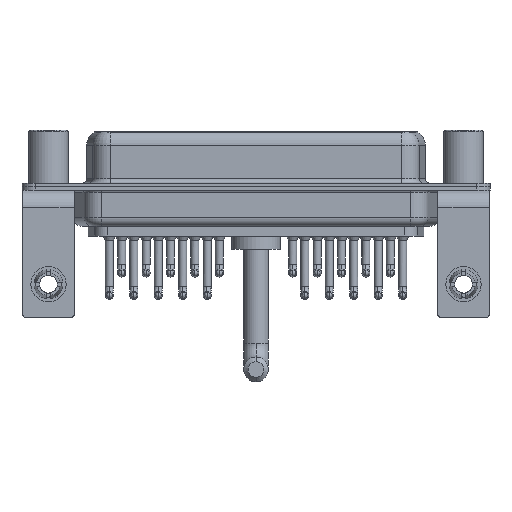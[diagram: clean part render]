
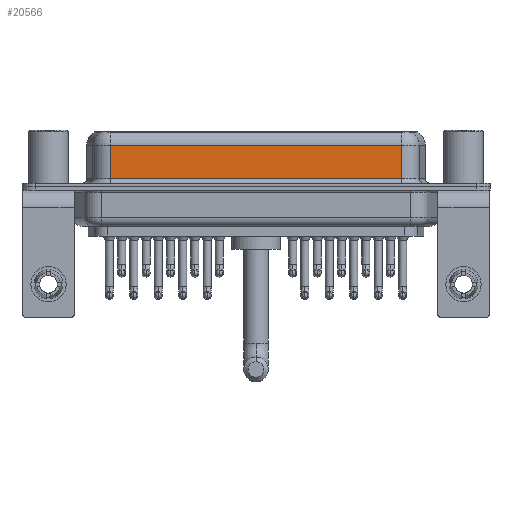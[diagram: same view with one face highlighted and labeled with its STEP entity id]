
A CAD part, front view. The second image highlights one B-rep face of the part: STEP entity #20566.
In plain terms, the highlighted planar face has unit normal (0, -1, 0).
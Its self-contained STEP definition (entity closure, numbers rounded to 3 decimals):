
#22 = DIRECTION ( 'NONE',  ( 0., 0., -1. ) ) ;
#668 = CARTESIAN_POINT ( 'NONE',  ( 40.037, -3.95, 4.65 ) ) ;
#1935 = DIRECTION ( 'NONE',  ( 0., 0., 1. ) ) ;
#2299 = LINE ( 'NONE', #668, #20552 ) ;
#2890 = VECTOR ( 'NONE', #9590, 1000. ) ;
#4066 = VECTOR ( 'NONE', #22, 1000. ) ;
#5206 = EDGE_CURVE ( 'NONE', #19438, #12582, #13756, .T. ) ;
#5814 = ORIENTED_EDGE ( 'NONE', *, *, #12244, .T. ) ;
#5881 = PLANE ( 'NONE',  #21403 ) ;
#9406 = VECTOR ( 'NONE', #24318, 1000. ) ;
#9524 = CARTESIAN_POINT ( 'NONE',  ( 40.037, -3.95, 0.9 ) ) ;
#9590 = DIRECTION ( 'NONE',  ( 0., 0., -1. ) ) ;
#9734 = LINE ( 'NONE', #14180, #2890 ) ;
#9865 = ORIENTED_EDGE ( 'NONE', *, *, #10973, .F. ) ;
#10973 = EDGE_CURVE ( 'NONE', #15545, #12582, #20626, .T. ) ;
#12244 = EDGE_CURVE ( 'NONE', #12977, #19438, #9734, .T. ) ;
#12582 = VERTEX_POINT ( 'NONE', #9524 ) ;
#12977 = VERTEX_POINT ( 'NONE', #15857 ) ;
#13756 = LINE ( 'NONE', #22438, #9406 ) ;
#13770 = ORIENTED_EDGE ( 'NONE', *, *, #5206, .T. ) ;
#14180 = CARTESIAN_POINT ( 'NONE',  ( 7.013, -3.95, 6.4 ) ) ;
#15545 = VERTEX_POINT ( 'NONE', #24174 ) ;
#15857 = CARTESIAN_POINT ( 'NONE',  ( 7.013, -3.95, 4.65 ) ) ;
#18470 = DIRECTION ( 'NONE',  ( 0., 1., 0. ) ) ;
#18867 = CARTESIAN_POINT ( 'NONE',  ( 7.013, -3.95, 0.9 ) ) ;
#19438 = VERTEX_POINT ( 'NONE', #18867 ) ;
#20497 = FACE_OUTER_BOUND ( 'NONE', #20662, .T. ) ;
#20552 = VECTOR ( 'NONE', #20862, 1000. ) ;
#20566 = ADVANCED_FACE ( 'NONE', ( #20497 ), #5881, .F. ) ;
#20626 = LINE ( 'NONE', #25087, #4066 ) ;
#20662 = EDGE_LOOP ( 'NONE', ( #9865, #20981, #5814, #13770 ) ) ;
#20862 = DIRECTION ( 'NONE',  ( -1., 0., 0. ) ) ;
#20895 = CARTESIAN_POINT ( 'NONE',  ( 40.037, -3.95, 6.4 ) ) ;
#20981 = ORIENTED_EDGE ( 'NONE', *, *, #21110, .T. ) ;
#21110 = EDGE_CURVE ( 'NONE', #15545, #12977, #2299, .T. ) ;
#21403 = AXIS2_PLACEMENT_3D ( 'NONE', #20895, #18470, #1935 ) ;
#22438 = CARTESIAN_POINT ( 'NONE',  ( 40.037, -3.95, 0.9 ) ) ;
#24174 = CARTESIAN_POINT ( 'NONE',  ( 40.037, -3.95, 4.65 ) ) ;
#24318 = DIRECTION ( 'NONE',  ( 1., 0., 0. ) ) ;
#25087 = CARTESIAN_POINT ( 'NONE',  ( 40.037, -3.95, 6.4 ) ) ;
